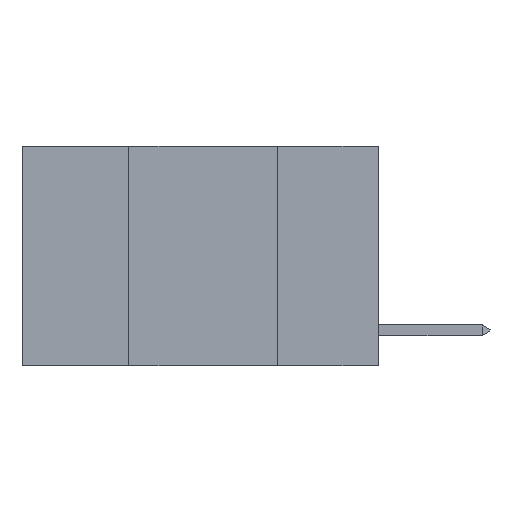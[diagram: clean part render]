
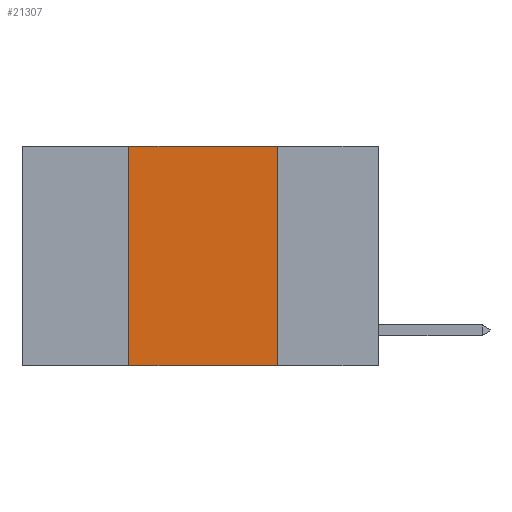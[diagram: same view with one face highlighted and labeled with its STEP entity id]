
A CAD part, left-side view. The second image highlights one B-rep face of the part: STEP entity #21307.
In plain terms, the highlighted planar face has unit normal (-1, 0, 0).
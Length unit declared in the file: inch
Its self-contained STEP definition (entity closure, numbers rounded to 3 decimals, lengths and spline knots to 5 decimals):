
#957 = FACE_OUTER_BOUND ( 'NONE', #17814, .T. ) ;
#1459 = VERTEX_POINT ( 'NONE', #11223 ) ;
#1516 = DIRECTION ( 'NONE',  ( 0., 0., 1. ) ) ;
#2008 = CARTESIAN_POINT ( 'NONE',  ( 0., 0.6, 0. ) ) ;
#2505 = VECTOR ( 'NONE', #8826, 39.37008 ) ;
#2573 = ORIENTED_EDGE ( 'NONE', *, *, #14251, .T. ) ;
#2661 = LINE ( 'NONE', #7744, #20474 ) ;
#2671 = PLANE ( 'NONE',  #7773 ) ;
#2826 = CARTESIAN_POINT ( 'NONE',  ( 0., 0.42, 0. ) ) ;
#3029 = ORIENTED_EDGE ( 'NONE', *, *, #3390, .F. ) ;
#3149 = LINE ( 'NONE', #2826, #11764 ) ;
#3390 = EDGE_CURVE ( 'NONE', #1459, #8412, #3149, .T. ) ;
#3502 = CARTESIAN_POINT ( 'NONE',  ( 0., 0.42, 0. ) ) ;
#4167 = CARTESIAN_POINT ( 'NONE',  ( 0., 0.17, -0.37 ) ) ;
#7102 = EDGE_CURVE ( 'NONE', #18775, #17204, #2661, .T. ) ;
#7555 = DIRECTION ( 'NONE',  ( 0., 0., -1. ) ) ;
#7744 = CARTESIAN_POINT ( 'NONE',  ( 0., 0.17, 0. ) ) ;
#7773 = AXIS2_PLACEMENT_3D ( 'NONE', #11120, #14368, #7555 ) ;
#8412 = VERTEX_POINT ( 'NONE', #3502 ) ;
#8826 = DIRECTION ( 'NONE',  ( 0., -1., 0. ) ) ;
#10338 = DIRECTION ( 'NONE',  ( 0., -1., 0. ) ) ;
#11120 = CARTESIAN_POINT ( 'NONE',  ( 0., 0.6, 0. ) ) ;
#11223 = CARTESIAN_POINT ( 'NONE',  ( 0., 0.42, -0.37 ) ) ;
#11764 = VECTOR ( 'NONE', #1516, 39.37008 ) ;
#11953 = CARTESIAN_POINT ( 'NONE',  ( 0., 0.17, 0. ) ) ;
#12306 = EDGE_CURVE ( 'NONE', #8412, #18775, #18462, .T. ) ;
#14133 = VECTOR ( 'NONE', #10338, 39.37008 ) ;
#14251 = EDGE_CURVE ( 'NONE', #1459, #17204, #17562, .T. ) ;
#14353 = DIRECTION ( 'NONE',  ( 0., 0., -1. ) ) ;
#14368 = DIRECTION ( 'NONE',  ( 1., 0., 0. ) ) ;
#15946 = CARTESIAN_POINT ( 'NONE',  ( 0., 0.6, -0.37 ) ) ;
#17204 = VERTEX_POINT ( 'NONE', #4167 ) ;
#17562 = LINE ( 'NONE', #15946, #2505 ) ;
#17814 = EDGE_LOOP ( 'NONE', ( #18337, #18676, #3029, #2573 ) ) ;
#18337 = ORIENTED_EDGE ( 'NONE', *, *, #7102, .F. ) ;
#18462 = LINE ( 'NONE', #2008, #14133 ) ;
#18676 = ORIENTED_EDGE ( 'NONE', *, *, #12306, .F. ) ;
#18775 = VERTEX_POINT ( 'NONE', #11953 ) ;
#20474 = VECTOR ( 'NONE', #14353, 39.37008 ) ;
#21307 = ADVANCED_FACE ( 'NONE', ( #957 ), #2671, .F. ) ;
